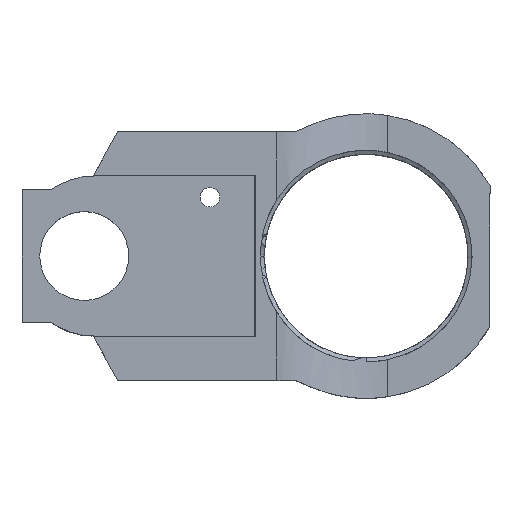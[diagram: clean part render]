
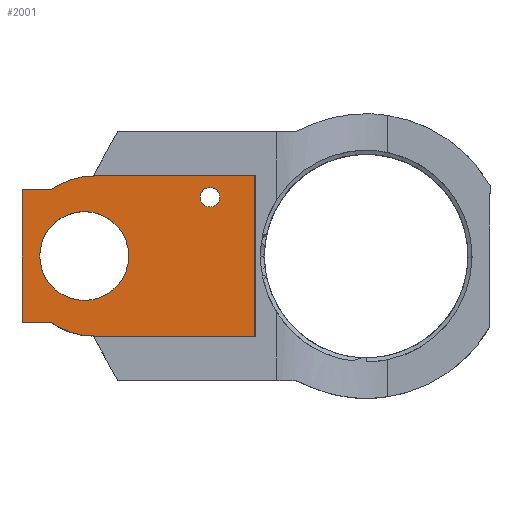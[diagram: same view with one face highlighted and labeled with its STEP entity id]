
A CAD part, top view. The second image highlights one B-rep face of the part: STEP entity #2001.
In plain terms, the highlighted planar face has unit normal (0, 0, 1).
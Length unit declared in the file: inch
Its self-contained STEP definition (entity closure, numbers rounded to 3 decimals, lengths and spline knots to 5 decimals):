
#84 = CARTESIAN_POINT ( 'NONE',  ( -4.37262, 2.9345, 0.30362 ) ) ;
#110 = LINE ( 'NONE', #5272, #5228 ) ;
#148 = EDGE_CURVE ( 'NONE', #2366, #4254, #2998, .T. ) ;
#204 = EDGE_CURVE ( 'NONE', #5511, #4359, #4560, .T. ) ;
#251 = CIRCLE ( 'NONE', #2961, 0.4 ) ;
#288 = AXIS2_PLACEMENT_3D ( 'NONE', #5250, #6117, #2604 ) ;
#370 = EDGE_CURVE ( 'NONE', #4254, #2366, #7909, .T. ) ;
#398 = ORIENTED_EDGE ( 'NONE', *, *, #2106, .T. ) ;
#547 = CARTESIAN_POINT ( 'NONE',  ( -3.41806, 2.2305, 0.30362 ) ) ;
#633 = CARTESIAN_POINT ( 'NONE',  ( -4.31986, 3.1385, 0.30362 ) ) ;
#782 = VERTEX_POINT ( 'NONE', #6077 ) ;
#811 = VERTEX_POINT ( 'NONE', #2713 ) ;
#815 = DIRECTION ( 'NONE',  ( -1., 0., 0. ) ) ;
#832 = CARTESIAN_POINT ( 'NONE',  ( -4.32262, 2.2355, 0.30362 ) ) ;
#1004 = VERTEX_POINT ( 'NONE', #547 ) ;
#1029 = CARTESIAN_POINT ( 'NONE',  ( -4.55631, 3.05813, 0.30362 ) ) ;
#1108 = VECTOR ( 'NONE', #3452, 39.37008 ) ;
#1140 = EDGE_LOOP ( 'NONE', ( #5608, #6894 ) ) ;
#1222 = EDGE_LOOP ( 'NONE', ( #8357, #398, #7281, #3946, #6234, #4671, #5588, #4477, #4230, #1618 ) ) ;
#1238 = CARTESIAN_POINT ( 'NONE',  ( -3.41162, 2.2305, 0.30362 ) ) ;
#1315 = FACE_BOUND ( 'NONE', #1140, .T. ) ;
#1430 = CARTESIAN_POINT ( 'NONE',  ( -4.32262, 2.7335, 0.30362 ) ) ;
#1481 = CARTESIAN_POINT ( 'NONE',  ( -3.66662, 3.015, 0.30362 ) ) ;
#1503 = ORIENTED_EDGE ( 'NONE', *, *, #148, .T. ) ;
#1541 = ORIENTED_EDGE ( 'NONE', *, *, #370, .T. ) ;
#1618 = ORIENTED_EDGE ( 'NONE', *, *, #6504, .F. ) ;
#1632 = CARTESIAN_POINT ( 'NONE',  ( -4.32262, 3.1335, 0.30362 ) ) ;
#1792 = CARTESIAN_POINT ( 'NONE',  ( -3.41806, 2.21636, 0.30362 ) ) ;
#1840 = DIRECTION ( 'NONE',  ( 0., 1., 0. ) ) ;
#1873 = DIRECTION ( 'NONE',  ( 1., 0., 0. ) ) ;
#1964 = EDGE_CURVE ( 'NONE', #7415, #1004, #7799, .T. ) ;
#2001 = ADVANCED_FACE ( 'NONE', ( #1315, #5485, #7379 ), #4791, .T. ) ;
#2058 = EDGE_CURVE ( 'NONE', #811, #3221, #6021, .T. ) ;
#2106 = EDGE_CURVE ( 'NONE', #2850, #811, #6857, .T. ) ;
#2290 = DIRECTION ( 'NONE',  ( -0.483, 0.875, 0. ) ) ;
#2300 = CARTESIAN_POINT ( 'NONE',  ( -4.37262, 2.6845, 0.30362 ) ) ;
#2366 = VERTEX_POINT ( 'NONE', #3140 ) ;
#2409 = VERTEX_POINT ( 'NONE', #633 ) ;
#2418 = AXIS2_PLACEMENT_3D ( 'NONE', #2300, #3636, #7681 ) ;
#2440 = DIRECTION ( 'NONE',  ( 1., 0., 0. ) ) ;
#2604 = DIRECTION ( 'NONE',  ( 1., 0., 0. ) ) ;
#2712 = EDGE_CURVE ( 'NONE', #7415, #7708, #6436, .T. ) ;
#2713 = CARTESIAN_POINT ( 'NONE',  ( -4.72262, 3.05813, 0.30362 ) ) ;
#2744 = EDGE_CURVE ( 'NONE', #7126, #2409, #4342, .T. ) ;
#2845 = DIRECTION ( 'NONE',  ( -1., 0., 0. ) ) ;
#2850 = VERTEX_POINT ( 'NONE', #1029 ) ;
#2900 = VERTEX_POINT ( 'NONE', #1632 ) ;
#2961 = AXIS2_PLACEMENT_3D ( 'NONE', #1430, #3442, #6838 ) ;
#2998 = CIRCLE ( 'NONE', #7072, 0.055 ) ;
#3140 = CARTESIAN_POINT ( 'NONE',  ( -3.66662, 2.96, 0.30362 ) ) ;
#3164 = AXIS2_PLACEMENT_3D ( 'NONE', #4512, #7738, #2440 ) ;
#3217 = CARTESIAN_POINT ( 'NONE',  ( -4.52262, 3.05813, 0.30362 ) ) ;
#3221 = VERTEX_POINT ( 'NONE', #6522 ) ;
#3442 = DIRECTION ( 'NONE',  ( 0., 0., -1. ) ) ;
#3452 = DIRECTION ( 'NONE',  ( -1., 0., 0. ) ) ;
#3492 = CARTESIAN_POINT ( 'NONE',  ( -4.52262, 2.31087, 0.30362 ) ) ;
#3528 = EDGE_CURVE ( 'NONE', #2850, #2900, #251, .T. ) ;
#3595 = DIRECTION ( 'NONE',  ( 1., 0., 0. ) ) ;
#3636 = DIRECTION ( 'NONE',  ( 0., 0., -1. ) ) ;
#3794 = VECTOR ( 'NONE', #1840, 39.37008 ) ;
#3946 = ORIENTED_EDGE ( 'NONE', *, *, #7206, .F. ) ;
#4230 = ORIENTED_EDGE ( 'NONE', *, *, #2744, .T. ) ;
#4232 = DIRECTION ( 'NONE',  ( 0., 0., -1. ) ) ;
#4243 = VECTOR ( 'NONE', #4761, 39.37008 ) ;
#4254 = VERTEX_POINT ( 'NONE', #8122 ) ;
#4277 = CARTESIAN_POINT ( 'NONE',  ( -4.18462, 1.9855, 0.30362 ) ) ;
#4342 = LINE ( 'NONE', #6848, #4645 ) ;
#4359 = VERTEX_POINT ( 'NONE', #6134 ) ;
#4477 = ORIENTED_EDGE ( 'NONE', *, *, #7287, .T. ) ;
#4512 = CARTESIAN_POINT ( 'NONE',  ( -4.32262, 2.6355, 0.30362 ) ) ;
#4560 = CIRCLE ( 'NONE', #2418, 0.25 ) ;
#4645 = VECTOR ( 'NONE', #2845, 39.37008 ) ;
#4667 = EDGE_CURVE ( 'NONE', #7708, #782, #5792, .T. ) ;
#4671 = ORIENTED_EDGE ( 'NONE', *, *, #2712, .F. ) ;
#4761 = DIRECTION ( 'NONE',  ( 0., -1., 0. ) ) ;
#4791 = PLANE ( 'NONE',  #288 ) ;
#4928 = CIRCLE ( 'NONE', #6706, 0.25 ) ;
#5228 = VECTOR ( 'NONE', #6610, 39.37008 ) ;
#5250 = CARTESIAN_POINT ( 'NONE',  ( -6.09162, 2.6845, 0.30362 ) ) ;
#5272 = CARTESIAN_POINT ( 'NONE',  ( -4.18462, 3.3835, 0.30362 ) ) ;
#5289 = EDGE_CURVE ( 'NONE', #4359, #5511, #4928, .T. ) ;
#5444 = CARTESIAN_POINT ( 'NONE',  ( -3.41806, 3.1385, 0.30362 ) ) ;
#5485 = FACE_OUTER_BOUND ( 'NONE', #1222, .T. ) ;
#5496 = EDGE_LOOP ( 'NONE', ( #1541, #1503 ) ) ;
#5511 = VERTEX_POINT ( 'NONE', #84 ) ;
#5544 = AXIS2_PLACEMENT_3D ( 'NONE', #5553, #7559, #3595 ) ;
#5553 = CARTESIAN_POINT ( 'NONE',  ( -3.66662, 3.015, 0.30362 ) ) ;
#5588 = ORIENTED_EDGE ( 'NONE', *, *, #1964, .T. ) ;
#5608 = ORIENTED_EDGE ( 'NONE', *, *, #204, .T. ) ;
#5792 = CIRCLE ( 'NONE', #3164, 0.4 ) ;
#6021 = LINE ( 'NONE', #6790, #4243 ) ;
#6077 = CARTESIAN_POINT ( 'NONE',  ( -4.55631, 2.31087, 0.30362 ) ) ;
#6117 = DIRECTION ( 'NONE',  ( 0., 0., 1. ) ) ;
#6134 = CARTESIAN_POINT ( 'NONE',  ( -4.37262, 2.4345, 0.30362 ) ) ;
#6234 = ORIENTED_EDGE ( 'NONE', *, *, #4667, .F. ) ;
#6436 = LINE ( 'NONE', #4277, #6752 ) ;
#6504 = EDGE_CURVE ( 'NONE', #2900, #2409, #110, .T. ) ;
#6522 = CARTESIAN_POINT ( 'NONE',  ( -4.72262, 2.31087, 0.30362 ) ) ;
#6610 = DIRECTION ( 'NONE',  ( 0.483, 0.875, 0. ) ) ;
#6653 = VECTOR ( 'NONE', #1873, 39.37008 ) ;
#6706 = AXIS2_PLACEMENT_3D ( 'NONE', #7959, #8644, #8523 ) ;
#6731 = VECTOR ( 'NONE', #815, 39.37008 ) ;
#6752 = VECTOR ( 'NONE', #2290, 39.37008 ) ;
#6790 = CARTESIAN_POINT ( 'NONE',  ( -4.72262, 3.1385, 0.30362 ) ) ;
#6838 = DIRECTION ( 'NONE',  ( 1., 0., 0. ) ) ;
#6848 = CARTESIAN_POINT ( 'NONE',  ( -3.41162, 3.1385, 0.30362 ) ) ;
#6857 = LINE ( 'NONE', #3217, #1108 ) ;
#6894 = ORIENTED_EDGE ( 'NONE', *, *, #5289, .T. ) ;
#7072 = AXIS2_PLACEMENT_3D ( 'NONE', #1481, #4232, #8266 ) ;
#7126 = VERTEX_POINT ( 'NONE', #5444 ) ;
#7206 = EDGE_CURVE ( 'NONE', #782, #3221, #8516, .T. ) ;
#7281 = ORIENTED_EDGE ( 'NONE', *, *, #2058, .T. ) ;
#7287 = EDGE_CURVE ( 'NONE', #1004, #7126, #7874, .T. ) ;
#7379 = FACE_BOUND ( 'NONE', #5496, .T. ) ;
#7415 = VERTEX_POINT ( 'NONE', #7985 ) ;
#7559 = DIRECTION ( 'NONE',  ( 0., 0., -1. ) ) ;
#7681 = DIRECTION ( 'NONE',  ( 1., 0., 0. ) ) ;
#7708 = VERTEX_POINT ( 'NONE', #832 ) ;
#7738 = DIRECTION ( 'NONE',  ( 0., 0., -1. ) ) ;
#7799 = LINE ( 'NONE', #1238, #6653 ) ;
#7874 = LINE ( 'NONE', #1792, #3794 ) ;
#7909 = CIRCLE ( 'NONE', #5544, 0.055 ) ;
#7959 = CARTESIAN_POINT ( 'NONE',  ( -4.37262, 2.6845, 0.30362 ) ) ;
#7985 = CARTESIAN_POINT ( 'NONE',  ( -4.31986, 2.2305, 0.30362 ) ) ;
#8122 = CARTESIAN_POINT ( 'NONE',  ( -3.66662, 3.07, 0.30362 ) ) ;
#8266 = DIRECTION ( 'NONE',  ( 1., 0., 0. ) ) ;
#8357 = ORIENTED_EDGE ( 'NONE', *, *, #3528, .F. ) ;
#8516 = LINE ( 'NONE', #3492, #6731 ) ;
#8523 = DIRECTION ( 'NONE',  ( 1., 0., 0. ) ) ;
#8644 = DIRECTION ( 'NONE',  ( 0., 0., -1. ) ) ;
